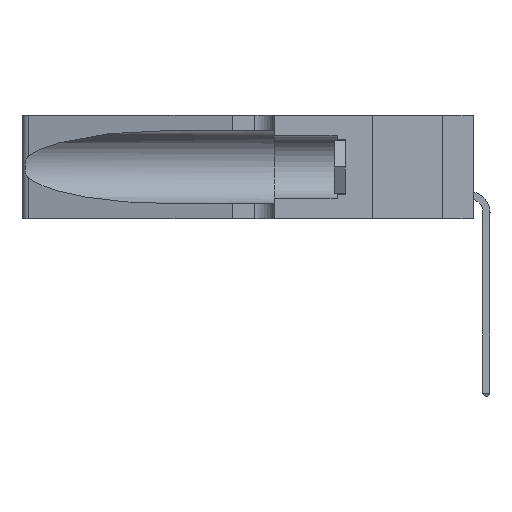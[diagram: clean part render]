
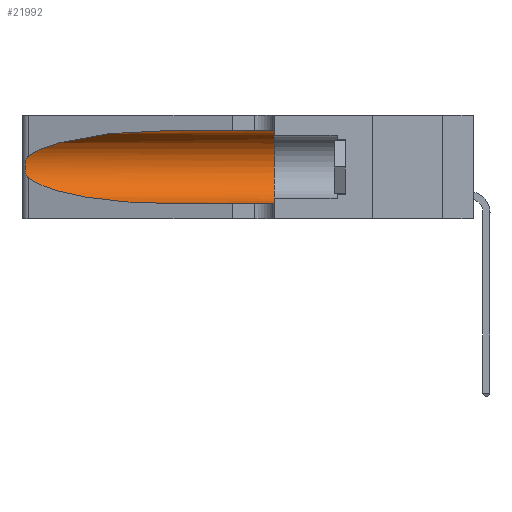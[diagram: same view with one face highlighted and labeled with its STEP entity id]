
A CAD part, left-side view. The second image highlights one B-rep face of the part: STEP entity #21992.
In plain terms, the highlighted cylindrical face has radius 3.308 mm (diameter 6.617 mm), a partial arc.
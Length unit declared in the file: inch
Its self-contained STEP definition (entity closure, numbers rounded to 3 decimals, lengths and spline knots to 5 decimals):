
#1393 = DIRECTION ( 'NONE',  ( 0., 1., 0. ) ) ;
#1464 = CARTESIAN_POINT ( 'NONE',  ( 0.25555, 1.22994, 0.2215 ) ) ;
#1483 = VECTOR ( 'NONE', #20245, 39.37008 ) ;
#1649 = CARTESIAN_POINT ( 'NONE',  ( 0.25639, 1.23186, 0.15144 ) ) ;
#1854 = CARTESIAN_POINT ( 'NONE',  ( 0.25856, 1.23593, 0.16098 ) ) ;
#1952 = CARTESIAN_POINT ( 'NONE',  ( 0.25789, 1.23486, 0.15765 ) ) ;
#2169 = VERTEX_POINT ( 'NONE', #17385 ) ;
#2618 = EDGE_CURVE ( 'NONE', #23729, #14149, #16596, .T. ) ;
#3721 = CARTESIAN_POINT ( 'NONE',  ( 0.25854, 1.2359, 0.20912 ) ) ;
#3843 = DIRECTION ( 'NONE',  ( 0., 0., 1. ) ) ;
#3849 = VERTEX_POINT ( 'NONE', #12783 ) ;
#3906 = EDGE_CURVE ( 'NONE', #14149, #3849, #26704, .T. ) ;
#3916 = CARTESIAN_POINT ( 'NONE',  ( 0.25555, 1.22993, 0.14849 ) ) ;
#4373 = ORIENTED_EDGE ( 'NONE', *, *, #3906, .F. ) ;
#4414 = CYLINDRICAL_SURFACE ( 'NONE', #11889, 0.13025 ) ;
#4641 = CARTESIAN_POINT ( 'NONE',  ( 0.1305, 0.35, 0.31525 ) ) ;
#5363 = CARTESIAN_POINT ( 'NONE',  ( 0.1305, 0.72297, 0.05475 ) ) ;
#5874 = EDGE_CURVE ( 'NONE', #2169, #10672, #18321, .T. ) ;
#5959 = CARTESIAN_POINT ( 'NONE',  ( 0.26018, 1.23835, 0.19895 ) ) ;
#6105 = EDGE_CURVE ( 'NONE', #10672, #10509, #24149, .T. ) ;
#6331 = CARTESIAN_POINT ( 'NONE',  ( 0.25487, 1.22718, 0.14631 ) ) ;
#6468 = DIRECTION ( 'NONE',  ( 0., -1., 0. ) ) ;
#7569 = DIRECTION ( 'NONE',  ( 0., -1., 0. ) ) ;
#7793 = ORIENTED_EDGE ( 'NONE', *, *, #8917, .T. ) ;
#8917 = EDGE_CURVE ( 'NONE', #23729, #2169, #21058, .T. ) ;
#9623 = CARTESIAN_POINT ( 'NONE',  ( 0.1305, 1.61858, 0.05475 ) ) ;
#9857 = CARTESIAN_POINT ( 'NONE',  ( 0.1305, 1.61858, 0.31525 ) ) ;
#10458 = ORIENTED_EDGE ( 'NONE', *, *, #2618, .F. ) ;
#10509 = VERTEX_POINT ( 'NONE', #18290 ) ;
#10608 = CARTESIAN_POINT ( 'NONE',  ( 0.26017, 1.23833, 0.17102 ) ) ;
#10672 = VERTEX_POINT ( 'NONE', #6331 ) ;
#11731 = EDGE_CURVE ( 'NONE', #10509, #3849, #19461, .T. ) ;
#11889 = AXIS2_PLACEMENT_3D ( 'NONE', #17561, #6468, #22209 ) ;
#12783 = CARTESIAN_POINT ( 'NONE',  ( 0.1305, 0.35, 0.05475 ) ) ;
#12839 = EDGE_LOOP ( 'NONE', ( #7793, #17647, #23401, #27862, #4373, #10458 ) ) ;
#12948 = CARTESIAN_POINT ( 'NONE',  ( 0.25487, 1.22718, 0.14631 ) ) ;
#13049 = CARTESIAN_POINT ( 'NONE',  ( 0.26075, 1.23896, 0.178 ) ) ;
#13648 = AXIS2_PLACEMENT_3D ( 'NONE', #17297, #1393, #3843 ) ;
#14149 = VERTEX_POINT ( 'NONE', #4641 ) ;
#14517 = CARTESIAN_POINT ( 'NONE',  ( 0.18966, 0.96281, 0.05475 ) ) ;
#14530 = CARTESIAN_POINT ( 'NONE',  ( 0.18966, 0.96281, 0.31525 ) ) ;
#14575 = VECTOR ( 'NONE', #7569, 39.37008 ) ;
#16069 = CARTESIAN_POINT ( 'NONE',  ( 0.2373, 1.15595, 0.08982 ) ) ;
#16596 = LINE ( 'NONE', #9857, #1483 ) ;
#17185 = CARTESIAN_POINT ( 'NONE',  ( 0.25787, 1.23484, 0.2124 ) ) ;
#17297 = CARTESIAN_POINT ( 'NONE',  ( 0.1305, 0.35, 0.185 ) ) ;
#17385 = CARTESIAN_POINT ( 'NONE',  ( 0.25487, 1.22718, 0.22369 ) ) ;
#17561 = CARTESIAN_POINT ( 'NONE',  ( 0.1305, 1.61858, 0.185 ) ) ;
#17647 = ORIENTED_EDGE ( 'NONE', *, *, #5874, .T. ) ;
#18290 = CARTESIAN_POINT ( 'NONE',  ( 0.1305, 0.72297, 0.05475 ) ) ;
#18321 = B_SPLINE_CURVE_WITH_KNOTS ( 'NONE', 3,
 ( #23689, #1464, #25908, #17185, #3721, #5959, #21702, #13049, #10608, #1854, #1952, #1649, #3916, #12948 ),
 .UNSPECIFIED., .F., .F.,
 ( 4, 2, 2, 2, 2, 2, 4 ),
 ( 0., 0.00027, 0.00053, 0.00107, 0.0016, 0.00187, 0.00214 ),
 .UNSPECIFIED. ) ;
#19461 = LINE ( 'NONE', #9623, #14575 ) ;
#20245 = DIRECTION ( 'NONE',  ( 0., -1., 0. ) ) ;
#21058 =( BOUNDED_CURVE ( )  B_SPLINE_CURVE ( 3, ( #23583, #14530, #27563, #27668 ),
 .UNSPECIFIED., .F., .T. ) 
 B_SPLINE_CURVE_WITH_KNOTS ( ( 4, 4 ),
 ( 1.5708, 2.84003 ),
 .UNSPECIFIED. ) 
 CURVE ( )  GEOMETRIC_REPRESENTATION_ITEM ( )  RATIONAL_B_SPLINE_CURVE ( ( 1., 0.87, 0.87, 1. ) ) 
 REPRESENTATION_ITEM ( '' )  );
#21321 = FACE_OUTER_BOUND ( 'NONE', #12839, .T. ) ;
#21702 = CARTESIAN_POINT ( 'NONE',  ( 0.26075, 1.23896, 0.19203 ) ) ;
#21992 = ADVANCED_FACE ( 'NONE', ( #21321 ), #4414, .F. ) ;
#22209 = DIRECTION ( 'NONE',  ( 0., 0., -1. ) ) ;
#23401 = ORIENTED_EDGE ( 'NONE', *, *, #6105, .T. ) ;
#23583 = CARTESIAN_POINT ( 'NONE',  ( 0.1305, 0.72297, 0.31525 ) ) ;
#23689 = CARTESIAN_POINT ( 'NONE',  ( 0.25487, 1.22718, 0.22369 ) ) ;
#23729 = VERTEX_POINT ( 'NONE', #25856 ) ;
#24149 =( BOUNDED_CURVE ( )  B_SPLINE_CURVE ( 3, ( #24921, #16069, #14517, #5363 ),
 .UNSPECIFIED., .F., .F. ) 
 B_SPLINE_CURVE_WITH_KNOTS ( ( 4, 4 ),
 ( 3.44316, 4.71239 ),
 .UNSPECIFIED. ) 
 CURVE ( )  GEOMETRIC_REPRESENTATION_ITEM ( )  RATIONAL_B_SPLINE_CURVE ( ( 1., 0.87, 0.87, 1. ) ) 
 REPRESENTATION_ITEM ( '' )  );
#24921 = CARTESIAN_POINT ( 'NONE',  ( 0.25487, 1.22718, 0.14631 ) ) ;
#25856 = CARTESIAN_POINT ( 'NONE',  ( 0.1305, 0.72297, 0.31525 ) ) ;
#25908 = CARTESIAN_POINT ( 'NONE',  ( 0.25639, 1.23184, 0.21858 ) ) ;
#26704 = CIRCLE ( 'NONE', #13648, 0.13025 ) ;
#27563 = CARTESIAN_POINT ( 'NONE',  ( 0.2373, 1.15595, 0.28018 ) ) ;
#27668 = CARTESIAN_POINT ( 'NONE',  ( 0.25487, 1.22718, 0.22369 ) ) ;
#27862 = ORIENTED_EDGE ( 'NONE', *, *, #11731, .T. ) ;
